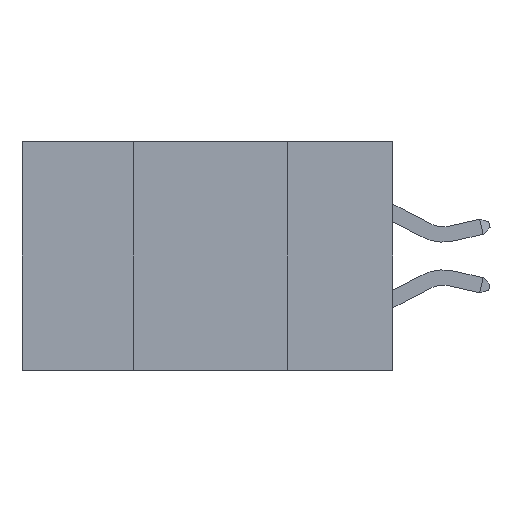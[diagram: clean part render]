
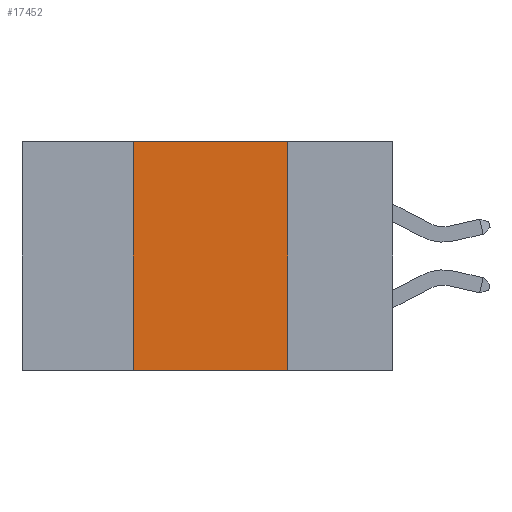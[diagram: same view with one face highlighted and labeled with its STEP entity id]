
A CAD part, left-side view. The second image highlights one B-rep face of the part: STEP entity #17452.
In plain terms, the highlighted planar face has unit normal (-1, 0, 0).
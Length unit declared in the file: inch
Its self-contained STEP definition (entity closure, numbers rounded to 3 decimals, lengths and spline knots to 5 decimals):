
#1183 = CARTESIAN_POINT ( 'NONE',  ( 0., 0.6, 0. ) ) ;
#1194 = VECTOR ( 'NONE', #29479, 39.37008 ) ;
#1403 = VERTEX_POINT ( 'NONE', #22263 ) ;
#4160 = ORIENTED_EDGE ( 'NONE', *, *, #25381, .F. ) ;
#5888 = VECTOR ( 'NONE', #18365, 39.37008 ) ;
#6880 = AXIS2_PLACEMENT_3D ( 'NONE', #19249, #25816, #31293 ) ;
#7359 = VERTEX_POINT ( 'NONE', #12170 ) ;
#8055 = DIRECTION ( 'NONE',  ( 0., -1., 0. ) ) ;
#8865 = CARTESIAN_POINT ( 'NONE',  ( 0., 0.17, 0. ) ) ;
#9246 = CARTESIAN_POINT ( 'NONE',  ( 0., 0.42, -0.37 ) ) ;
#9253 = FACE_OUTER_BOUND ( 'NONE', #23264, .T. ) ;
#9382 = CARTESIAN_POINT ( 'NONE',  ( 0., 0.42, 0. ) ) ;
#10555 = CARTESIAN_POINT ( 'NONE',  ( 0., 0.17, -0.37 ) ) ;
#12085 = ORIENTED_EDGE ( 'NONE', *, *, #18820, .F. ) ;
#12170 = CARTESIAN_POINT ( 'NONE',  ( 0., 0.42, 0. ) ) ;
#13667 = EDGE_CURVE ( 'NONE', #25552, #19524, #24940, .T. ) ;
#15529 = DIRECTION ( 'NONE',  ( 0., -1., 0. ) ) ;
#16417 = LINE ( 'NONE', #8865, #5888 ) ;
#17105 = LINE ( 'NONE', #9382, #1194 ) ;
#17361 = VECTOR ( 'NONE', #15529, 39.37008 ) ;
#17452 = ADVANCED_FACE ( 'NONE', ( #9253 ), #21172, .F. ) ;
#18365 = DIRECTION ( 'NONE',  ( 0., 0., -1. ) ) ;
#18389 = EDGE_CURVE ( 'NONE', #1403, #19524, #16417, .T. ) ;
#18428 = LINE ( 'NONE', #1183, #17361 ) ;
#18820 = EDGE_CURVE ( 'NONE', #25552, #7359, #17105, .T. ) ;
#19249 = CARTESIAN_POINT ( 'NONE',  ( 0., 0.6, 0. ) ) ;
#19524 = VERTEX_POINT ( 'NONE', #10555 ) ;
#20345 = ORIENTED_EDGE ( 'NONE', *, *, #13667, .T. ) ;
#21172 = PLANE ( 'NONE',  #6880 ) ;
#22263 = CARTESIAN_POINT ( 'NONE',  ( 0., 0.17, 0. ) ) ;
#23264 = EDGE_LOOP ( 'NONE', ( #27760, #4160, #12085, #20345 ) ) ;
#24940 = LINE ( 'NONE', #25570, #27756 ) ;
#25381 = EDGE_CURVE ( 'NONE', #7359, #1403, #18428, .T. ) ;
#25552 = VERTEX_POINT ( 'NONE', #9246 ) ;
#25570 = CARTESIAN_POINT ( 'NONE',  ( 0., 0.6, -0.37 ) ) ;
#25816 = DIRECTION ( 'NONE',  ( 1., 0., 0. ) ) ;
#27756 = VECTOR ( 'NONE', #8055, 39.37008 ) ;
#27760 = ORIENTED_EDGE ( 'NONE', *, *, #18389, .F. ) ;
#29479 = DIRECTION ( 'NONE',  ( 0., 0., 1. ) ) ;
#31293 = DIRECTION ( 'NONE',  ( 0., 0., -1. ) ) ;
